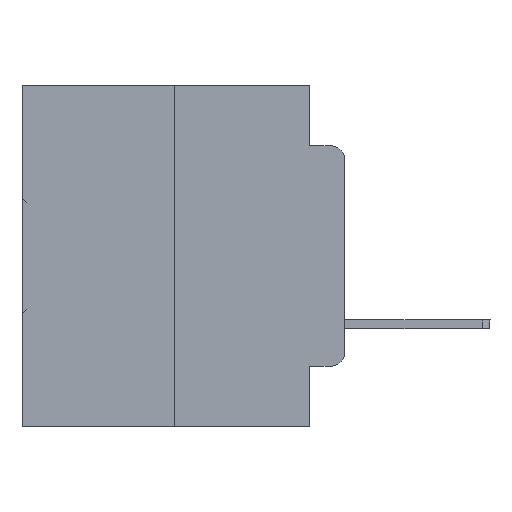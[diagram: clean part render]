
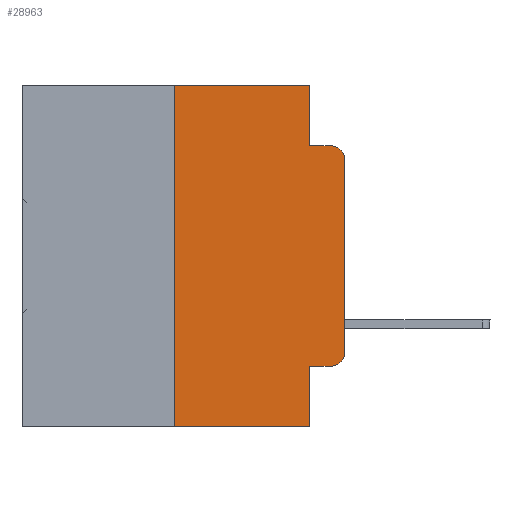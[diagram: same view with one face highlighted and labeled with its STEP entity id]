
A CAD part, left-side view. The second image highlights one B-rep face of the part: STEP entity #28963.
In plain terms, the highlighted planar face has unit normal (-1, 0, 0).
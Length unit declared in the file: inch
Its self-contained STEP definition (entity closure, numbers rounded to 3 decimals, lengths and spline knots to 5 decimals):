
#357 = LINE ( 'NONE', #12821, #23773 ) ;
#485 = VERTEX_POINT ( 'NONE', #5323 ) ;
#1501 = DIRECTION ( 'NONE',  ( 0., 0., -1. ) ) ;
#1599 = AXIS2_PLACEMENT_3D ( 'NONE', #23760, #31566, #16138 ) ;
#1655 = LINE ( 'NONE', #4770, #3644 ) ;
#1863 = ORIENTED_EDGE ( 'NONE', *, *, #8754, .F. ) ;
#1995 = ORIENTED_EDGE ( 'NONE', *, *, #17385, .T. ) ;
#2021 = CARTESIAN_POINT ( 'NONE',  ( 0., 0.051, -0.4115 ) ) ;
#2794 = VERTEX_POINT ( 'NONE', #9282 ) ;
#3024 = ORIENTED_EDGE ( 'NONE', *, *, #3888, .T. ) ;
#3035 = PLANE ( 'NONE',  #10100 ) ;
#3143 = CARTESIAN_POINT ( 'NONE',  ( 0., 0.051, 0. ) ) ;
#3161 = LINE ( 'NONE', #3143, #6878 ) ;
#3644 = VECTOR ( 'NONE', #28210, 39.37008 ) ;
#3888 = EDGE_CURVE ( 'NONE', #27433, #31271, #1655, .T. ) ;
#4702 = EDGE_CURVE ( 'NONE', #2794, #17276, #357, .T. ) ;
#4770 = CARTESIAN_POINT ( 'NONE',  ( 0., 0.051, -0.4115 ) ) ;
#4818 = CARTESIAN_POINT ( 'NONE',  ( 0., 0.25, 0. ) ) ;
#4819 = EDGE_CURVE ( 'NONE', #31271, #7744, #8065, .T. ) ;
#5323 = CARTESIAN_POINT ( 'NONE',  ( 0., 0.051, -0.5 ) ) ;
#6154 = ORIENTED_EDGE ( 'NONE', *, *, #23815, .T. ) ;
#6605 = LINE ( 'NONE', #17088, #10645 ) ;
#6744 = DIRECTION ( 'NONE',  ( -1., 0., 0. ) ) ;
#6878 = VECTOR ( 'NONE', #28893, 39.37008 ) ;
#6907 = VECTOR ( 'NONE', #22856, 39.37008 ) ;
#7744 = VERTEX_POINT ( 'NONE', #16315 ) ;
#8065 = CIRCLE ( 'NONE', #1599, 0.02 ) ;
#8754 = EDGE_CURVE ( 'NONE', #27433, #485, #18859, .T. ) ;
#9282 = CARTESIAN_POINT ( 'NONE',  ( 0., 0.051, -0.0885 ) ) ;
#10001 = ORIENTED_EDGE ( 'NONE', *, *, #4819, .T. ) ;
#10100 = AXIS2_PLACEMENT_3D ( 'NONE', #10869, #31486, #16059 ) ;
#10177 = DIRECTION ( 'NONE',  ( 0., 0., -1. ) ) ;
#10265 = ORIENTED_EDGE ( 'NONE', *, *, #31388, .F. ) ;
#10438 = EDGE_CURVE ( 'NONE', #25680, #485, #30469, .T. ) ;
#10645 = VECTOR ( 'NONE', #11449, 39.37008 ) ;
#10869 = CARTESIAN_POINT ( 'NONE',  ( 0., 0.473, 0. ) ) ;
#11449 = DIRECTION ( 'NONE',  ( 0., -1., 0. ) ) ;
#11733 = ORIENTED_EDGE ( 'NONE', *, *, #31592, .F. ) ;
#12085 = CARTESIAN_POINT ( 'NONE',  ( 0., 0.02, -0.4115 ) ) ;
#12602 = DIRECTION ( 'NONE',  ( 0., -1., 0. ) ) ;
#12821 = CARTESIAN_POINT ( 'NONE',  ( 0., 0.051, -0.0885 ) ) ;
#13529 = VERTEX_POINT ( 'NONE', #21036 ) ;
#13565 = CIRCLE ( 'NONE', #13653, 0.02 ) ;
#13581 = ORIENTED_EDGE ( 'NONE', *, *, #10438, .T. ) ;
#13653 = AXIS2_PLACEMENT_3D ( 'NONE', #22164, #6744, #1501 ) ;
#15123 = FACE_OUTER_BOUND ( 'NONE', #20534, .T. ) ;
#15172 = CARTESIAN_POINT ( 'NONE',  ( 0., 0., -0.1085 ) ) ;
#15183 = DIRECTION ( 'NONE',  ( 0., -1., 0. ) ) ;
#15394 = CARTESIAN_POINT ( 'NONE',  ( 0., 0.25, -0.5 ) ) ;
#15447 = VECTOR ( 'NONE', #26598, 39.37008 ) ;
#15562 = VECTOR ( 'NONE', #15183, 39.37008 ) ;
#16032 = CARTESIAN_POINT ( 'NONE',  ( 0., 0., 0. ) ) ;
#16059 = DIRECTION ( 'NONE',  ( 0., 0., -1. ) ) ;
#16138 = DIRECTION ( 'NONE',  ( 0., 0., -1. ) ) ;
#16315 = CARTESIAN_POINT ( 'NONE',  ( 0., 0., -0.3915 ) ) ;
#17088 = CARTESIAN_POINT ( 'NONE',  ( 0., 0.473, 0. ) ) ;
#17276 = VERTEX_POINT ( 'NONE', #22785 ) ;
#17385 = EDGE_CURVE ( 'NONE', #7744, #25863, #24225, .T. ) ;
#17810 = CARTESIAN_POINT ( 'NONE',  ( 0., 0.051, 0. ) ) ;
#18859 = LINE ( 'NONE', #30898, #20105 ) ;
#20105 = VECTOR ( 'NONE', #10177, 39.37008 ) ;
#20534 = EDGE_LOOP ( 'NONE', ( #1995, #6154, #21220, #11733, #21723, #10265, #13581, #1863, #3024, #10001 ) ) ;
#21036 = CARTESIAN_POINT ( 'NONE',  ( 0., 0.25, 0. ) ) ;
#21220 = ORIENTED_EDGE ( 'NONE', *, *, #4702, .F. ) ;
#21373 = LINE ( 'NONE', #4818, #6907 ) ;
#21723 = ORIENTED_EDGE ( 'NONE', *, *, #29009, .F. ) ;
#22164 = CARTESIAN_POINT ( 'NONE',  ( 0., 0.02, -0.1085 ) ) ;
#22785 = CARTESIAN_POINT ( 'NONE',  ( 0., 0.02, -0.0885 ) ) ;
#22856 = DIRECTION ( 'NONE',  ( 0., 0., 1. ) ) ;
#23760 = CARTESIAN_POINT ( 'NONE',  ( 0., 0.02, -0.3915 ) ) ;
#23773 = VECTOR ( 'NONE', #12602, 39.37008 ) ;
#23815 = EDGE_CURVE ( 'NONE', #25863, #17276, #13565, .T. ) ;
#24225 = LINE ( 'NONE', #16032, #15447 ) ;
#25680 = VERTEX_POINT ( 'NONE', #15394 ) ;
#25863 = VERTEX_POINT ( 'NONE', #15172 ) ;
#26598 = DIRECTION ( 'NONE',  ( 0., 0., 1. ) ) ;
#27433 = VERTEX_POINT ( 'NONE', #2021 ) ;
#28210 = DIRECTION ( 'NONE',  ( 0., -1., 0. ) ) ;
#28893 = DIRECTION ( 'NONE',  ( 0., 0., -1. ) ) ;
#28963 = ADVANCED_FACE ( 'NONE', ( #15123 ), #3035, .F. ) ;
#29009 = EDGE_CURVE ( 'NONE', #13529, #30894, #6605, .T. ) ;
#30469 = LINE ( 'NONE', #33291, #15562 ) ;
#30894 = VERTEX_POINT ( 'NONE', #17810 ) ;
#30898 = CARTESIAN_POINT ( 'NONE',  ( 0., 0.051, 0. ) ) ;
#31271 = VERTEX_POINT ( 'NONE', #12085 ) ;
#31388 = EDGE_CURVE ( 'NONE', #25680, #13529, #21373, .T. ) ;
#31486 = DIRECTION ( 'NONE',  ( 1., 0., 0. ) ) ;
#31566 = DIRECTION ( 'NONE',  ( -1., 0., 0. ) ) ;
#31592 = EDGE_CURVE ( 'NONE', #30894, #2794, #3161, .T. ) ;
#33291 = CARTESIAN_POINT ( 'NONE',  ( 0., 0.473, -0.5 ) ) ;
